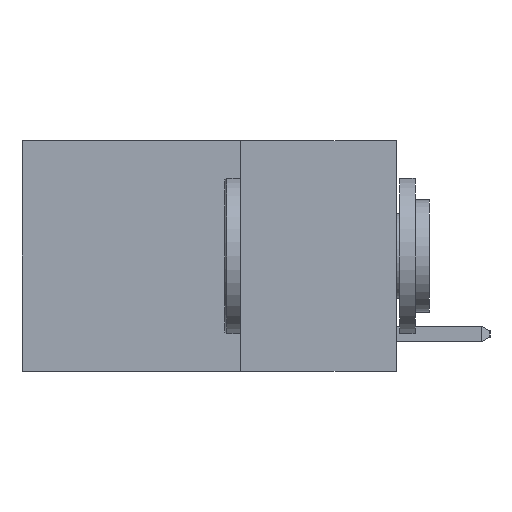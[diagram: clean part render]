
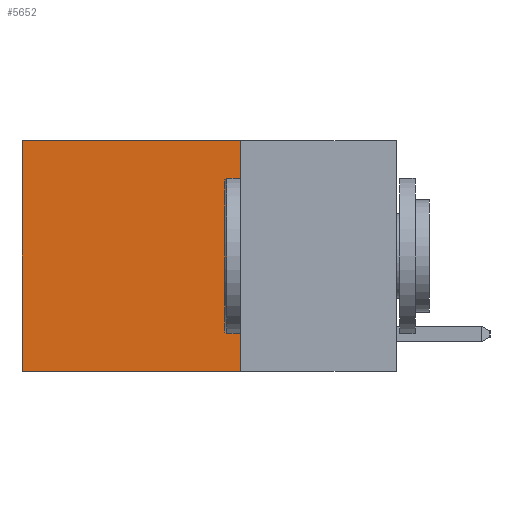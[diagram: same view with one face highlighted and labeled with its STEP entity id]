
A CAD part, left-side view. The second image highlights one B-rep face of the part: STEP entity #5652.
In plain terms, the highlighted planar face has unit normal (-1, 0, 0).
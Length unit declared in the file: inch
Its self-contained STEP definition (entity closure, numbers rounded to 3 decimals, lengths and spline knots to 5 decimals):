
#137 = CARTESIAN_POINT ( 'NONE',  ( 0.2625, 0.25, 0. ) ) ;
#210 = EDGE_CURVE ( 'NONE', #951, #2212, #7823, .T. ) ;
#618 = VECTOR ( 'NONE', #9300, 39.37008 ) ;
#684 = DIRECTION ( 'NONE',  ( 0., 1., 0. ) ) ;
#951 = VERTEX_POINT ( 'NONE', #11656 ) ;
#1499 = VECTOR ( 'NONE', #5384, 39.37008 ) ;
#1518 = DIRECTION ( 'NONE',  ( 1., 0., 0. ) ) ;
#2212 = VERTEX_POINT ( 'NONE', #4093 ) ;
#2367 = ORIENTED_EDGE ( 'NONE', *, *, #11061, .T. ) ;
#2884 = ORIENTED_EDGE ( 'NONE', *, *, #210, .F. ) ;
#2990 = DIRECTION ( 'NONE',  ( 0., 0., -1. ) ) ;
#3259 = ORIENTED_EDGE ( 'NONE', *, *, #8211, .F. ) ;
#3797 = LINE ( 'NONE', #137, #6258 ) ;
#4005 = LINE ( 'NONE', #8148, #1499 ) ;
#4093 = CARTESIAN_POINT ( 'NONE',  ( 0.2625, 0.6, -0.37 ) ) ;
#5384 = DIRECTION ( 'NONE',  ( 0., 0., -1. ) ) ;
#5472 = CARTESIAN_POINT ( 'NONE',  ( 0.2625, 0.25, 0. ) ) ;
#5652 = ADVANCED_FACE ( 'NONE', ( #12042 ), #7107, .F. ) ;
#5726 = EDGE_CURVE ( 'NONE', #10081, #2212, #4005, .T. ) ;
#6194 = VERTEX_POINT ( 'NONE', #5472 ) ;
#6258 = VECTOR ( 'NONE', #2990, 39.37008 ) ;
#6751 = CARTESIAN_POINT ( 'NONE',  ( 0.2625, 0.6, 0. ) ) ;
#7107 = PLANE ( 'NONE',  #7876 ) ;
#7335 = CARTESIAN_POINT ( 'NONE',  ( 0.2625, 0.25, -0.37 ) ) ;
#7466 = ORIENTED_EDGE ( 'NONE', *, *, #5726, .T. ) ;
#7823 = LINE ( 'NONE', #7335, #618 ) ;
#7876 = AXIS2_PLACEMENT_3D ( 'NONE', #8976, #1518, #8071 ) ;
#8071 = DIRECTION ( 'NONE',  ( 0., 0., -1. ) ) ;
#8148 = CARTESIAN_POINT ( 'NONE',  ( 0.2625, 0.6, 0. ) ) ;
#8211 = EDGE_CURVE ( 'NONE', #6194, #951, #3797, .T. ) ;
#8368 = EDGE_LOOP ( 'NONE', ( #7466, #2884, #3259, #2367 ) ) ;
#8976 = CARTESIAN_POINT ( 'NONE',  ( 0.2625, 0.25, 0. ) ) ;
#9300 = DIRECTION ( 'NONE',  ( 0., 1., 0. ) ) ;
#10081 = VERTEX_POINT ( 'NONE', #6751 ) ;
#11061 = EDGE_CURVE ( 'NONE', #6194, #10081, #11416, .T. ) ;
#11127 = VECTOR ( 'NONE', #684, 39.37008 ) ;
#11416 = LINE ( 'NONE', #11940, #11127 ) ;
#11656 = CARTESIAN_POINT ( 'NONE',  ( 0.2625, 0.25, -0.37 ) ) ;
#11940 = CARTESIAN_POINT ( 'NONE',  ( 0.2625, 0.25, 0. ) ) ;
#12042 = FACE_OUTER_BOUND ( 'NONE', #8368, .T. ) ;
